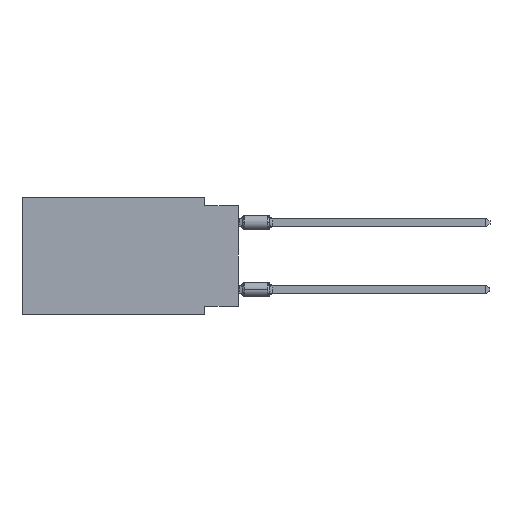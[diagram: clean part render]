
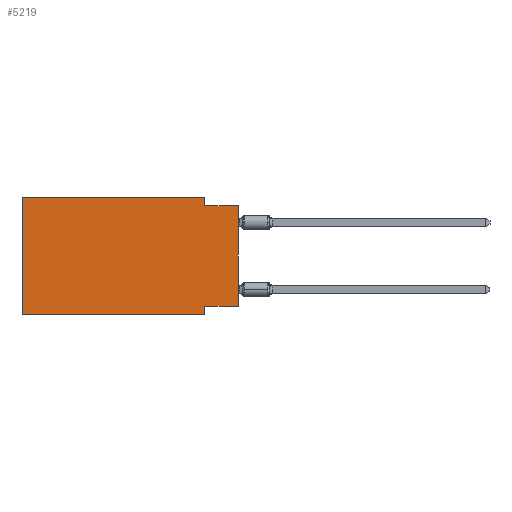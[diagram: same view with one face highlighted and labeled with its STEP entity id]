
A CAD part, left-side view. The second image highlights one B-rep face of the part: STEP entity #5219.
In plain terms, the highlighted planar face has unit normal (-1, 0, 0).
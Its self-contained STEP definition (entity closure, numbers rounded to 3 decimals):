
#372 = FACE_OUTER_BOUND ( 'NONE', #16579, .T. ) ;
#1187 = ORIENTED_EDGE ( 'NONE', *, *, #11656, .F. ) ;
#1401 = CARTESIAN_POINT ( 'NONE',  ( 0., 2.54, -8.255 ) ) ;
#2104 = ORIENTED_EDGE ( 'NONE', *, *, #3843, .F. ) ;
#2415 = VECTOR ( 'NONE', #7769, 1000. ) ;
#2546 = VERTEX_POINT ( 'NONE', #7097 ) ;
#2664 = CARTESIAN_POINT ( 'NONE',  ( 0., 0., -8.255 ) ) ;
#2793 = CARTESIAN_POINT ( 'NONE',  ( 0., 2.54, 0. ) ) ;
#2827 = VERTEX_POINT ( 'NONE', #3013 ) ;
#2895 = VERTEX_POINT ( 'NONE', #1401 ) ;
#2959 = VECTOR ( 'NONE', #10146, 1000. ) ;
#3013 = CARTESIAN_POINT ( 'NONE',  ( 0., 16.383, 0. ) ) ;
#3710 = CARTESIAN_POINT ( 'NONE',  ( 0., 0., 0. ) ) ;
#3840 = EDGE_CURVE ( 'NONE', #15092, #2827, #12782, .T. ) ;
#3843 = EDGE_CURVE ( 'NONE', #13092, #14035, #15327, .T. ) ;
#4115 = CARTESIAN_POINT ( 'NONE',  ( 0., 16.383, 0. ) ) ;
#4121 = CARTESIAN_POINT ( 'NONE',  ( 0., 16.383, -8.89 ) ) ;
#4178 = VECTOR ( 'NONE', #14260, 1000. ) ;
#5219 = ADVANCED_FACE ( 'NONE', ( #372 ), #12082, .F. ) ;
#5478 = CARTESIAN_POINT ( 'NONE',  ( 0., 0., -8.255 ) ) ;
#5687 = LINE ( 'NONE', #10859, #9768 ) ;
#6331 = DIRECTION ( 'NONE',  ( 0., 0., 1. ) ) ;
#6334 = VERTEX_POINT ( 'NONE', #13819 ) ;
#6591 = VERTEX_POINT ( 'NONE', #5478 ) ;
#6641 = DIRECTION ( 'NONE',  ( 0., 1., 0. ) ) ;
#6744 = DIRECTION ( 'NONE',  ( 0., 0., -1. ) ) ;
#7097 = CARTESIAN_POINT ( 'NONE',  ( 0., 2.54, -8.89 ) ) ;
#7456 = ORIENTED_EDGE ( 'NONE', *, *, #3840, .F. ) ;
#7717 = LINE ( 'NONE', #11774, #12978 ) ;
#7765 = AXIS2_PLACEMENT_3D ( 'NONE', #4115, #14559, #6744 ) ;
#7769 = DIRECTION ( 'NONE',  ( 0., 0., -1. ) ) ;
#8426 = VECTOR ( 'NONE', #6331, 1000. ) ;
#8783 = CARTESIAN_POINT ( 'NONE',  ( 0., 16.383, 0. ) ) ;
#8880 = ORIENTED_EDGE ( 'NONE', *, *, #11021, .T. ) ;
#9077 = CARTESIAN_POINT ( 'NONE',  ( 0., 0., -0.635 ) ) ;
#9609 = LINE ( 'NONE', #13608, #14120 ) ;
#9716 = ORIENTED_EDGE ( 'NONE', *, *, #15613, .T. ) ;
#9768 = VECTOR ( 'NONE', #16127, 1000. ) ;
#10146 = DIRECTION ( 'NONE',  ( 0., 0., 1. ) ) ;
#10859 = CARTESIAN_POINT ( 'NONE',  ( 0., 16.383, 0. ) ) ;
#11021 = EDGE_CURVE ( 'NONE', #6591, #6334, #15505, .T. ) ;
#11656 = EDGE_CURVE ( 'NONE', #2827, #13092, #5687, .T. ) ;
#11657 = LINE ( 'NONE', #2664, #13263 ) ;
#11774 = CARTESIAN_POINT ( 'NONE',  ( 0., 2.54, -8.89 ) ) ;
#12082 = PLANE ( 'NONE',  #7765 ) ;
#12158 = DIRECTION ( 'NONE',  ( 0., -1., 0. ) ) ;
#12565 = CARTESIAN_POINT ( 'NONE',  ( 0., 2.54, -0.635 ) ) ;
#12782 = LINE ( 'NONE', #8783, #2959 ) ;
#12978 = VECTOR ( 'NONE', #15783, 1000. ) ;
#13076 = EDGE_CURVE ( 'NONE', #2895, #2546, #7717, .T. ) ;
#13092 = VERTEX_POINT ( 'NONE', #2793 ) ;
#13263 = VECTOR ( 'NONE', #6641, 1000. ) ;
#13608 = CARTESIAN_POINT ( 'NONE',  ( 0., 16.383, -8.89 ) ) ;
#13819 = CARTESIAN_POINT ( 'NONE',  ( 0., 0., -0.635 ) ) ;
#14035 = VERTEX_POINT ( 'NONE', #12565 ) ;
#14120 = VECTOR ( 'NONE', #12158, 1000. ) ;
#14260 = DIRECTION ( 'NONE',  ( 0., -1., 0. ) ) ;
#14297 = EDGE_CURVE ( 'NONE', #6591, #2895, #11657, .T. ) ;
#14424 = LINE ( 'NONE', #9077, #4178 ) ;
#14482 = ORIENTED_EDGE ( 'NONE', *, *, #16298, .F. ) ;
#14559 = DIRECTION ( 'NONE',  ( 1., 0., 0. ) ) ;
#15092 = VERTEX_POINT ( 'NONE', #4121 ) ;
#15327 = LINE ( 'NONE', #15413, #2415 ) ;
#15413 = CARTESIAN_POINT ( 'NONE',  ( 0., 2.54, 0. ) ) ;
#15505 = LINE ( 'NONE', #3710, #8426 ) ;
#15613 = EDGE_CURVE ( 'NONE', #15092, #2546, #9609, .T. ) ;
#15783 = DIRECTION ( 'NONE',  ( 0., 0., -1. ) ) ;
#16127 = DIRECTION ( 'NONE',  ( 0., -1., 0. ) ) ;
#16298 = EDGE_CURVE ( 'NONE', #14035, #6334, #14424, .T. ) ;
#16430 = ORIENTED_EDGE ( 'NONE', *, *, #14297, .F. ) ;
#16492 = ORIENTED_EDGE ( 'NONE', *, *, #13076, .F. ) ;
#16579 = EDGE_LOOP ( 'NONE', ( #8880, #14482, #2104, #1187, #7456, #9716, #16492, #16430 ) ) ;
